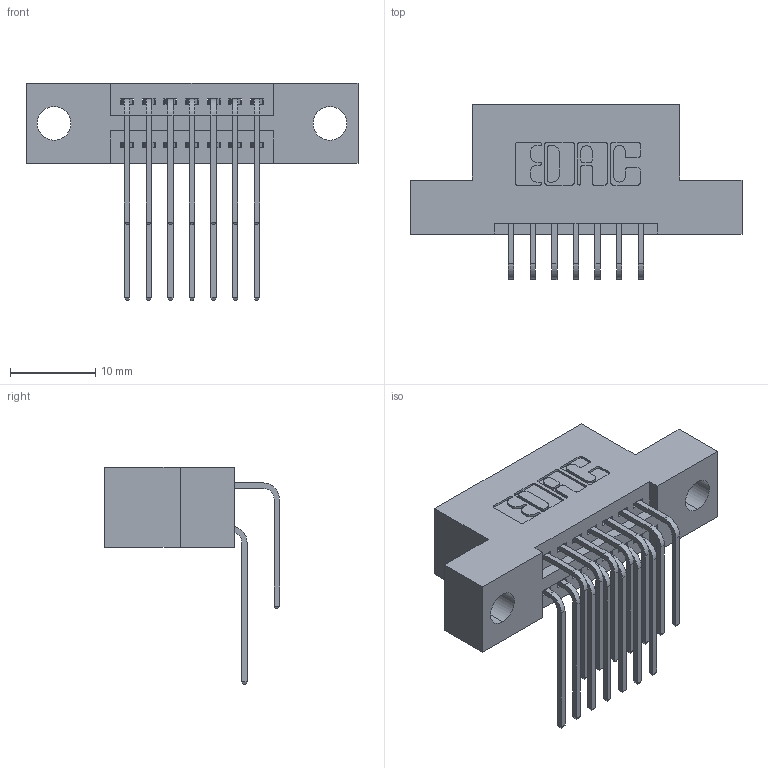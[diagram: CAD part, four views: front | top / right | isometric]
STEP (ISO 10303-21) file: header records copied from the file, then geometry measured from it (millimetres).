
FILE_DESCRIPTION (( 'STEP AP203' ), '1' );
FILE_NAME ('345-014-559-204.STEP', '2021-05-19T16:09:12', ( '' ), ( '' ), 'SwSTEP 2.0', 'SolidWorks 2020', '' );
FILE_SCHEMA (( 'CONFIG_CONTROL_DESIGN' ));
Length unit declared in the file: inch
Products named in the file (4): 345 Part_Flush Mounting Lugs - 0.156 Dia-TI; 345-292-001_559 Tail - 2; 345-014-559-204; 345-292-001_558 559 Tail - 1
Assembly tree (15 placements, depth 2):
  345-014-559-204
    345 Part_Flush Mounting Lugs - 0.156 Dia-TI
    345-292-001_558 559 Tail - 1  x7
    345-292-001_559 Tail - 2  x7
Bounding box: 38.99 x 20.56 x 25.53 mm (x, y, z)
Volume: 3437.4 mm3; surface area: 4634.5 mm2
Topology: 15 solids, 15 shells, 868 faces, 2547 edges, 1678 vertices
Faces by surface type: plane 584, cylinder 284
Entity records: 12275 total; most frequent: CARTESIAN_POINT 2141, ORIENTED_EDGE 2022, DIRECTION 1903, EDGE_CURVE 1011, LINE 811, VECTOR 811, VERTEX_POINT 670, AXIS2_PLACEMENT_3D 546
